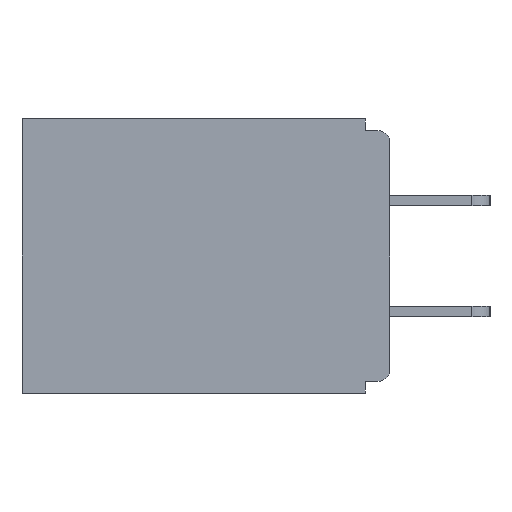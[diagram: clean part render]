
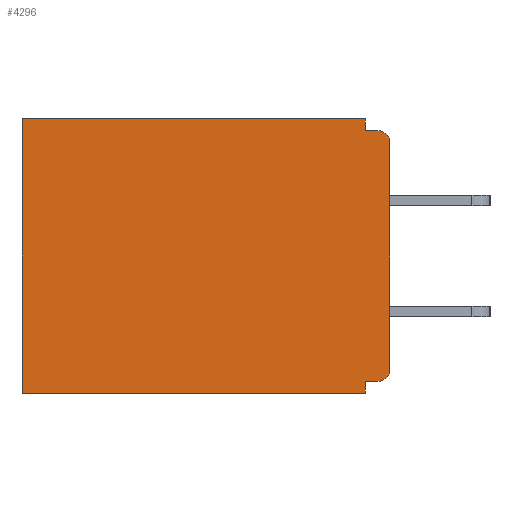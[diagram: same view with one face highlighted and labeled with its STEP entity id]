
A CAD part, left-side view. The second image highlights one B-rep face of the part: STEP entity #4296.
In plain terms, the highlighted planar face has unit normal (-1, 0, 0).
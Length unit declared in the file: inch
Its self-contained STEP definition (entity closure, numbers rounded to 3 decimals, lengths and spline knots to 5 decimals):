
#101 = CARTESIAN_POINT ( 'NONE',  ( 0.298, 0., -0.015 ) ) ;
#602 = LINE ( 'NONE', #17023, #18324 ) ;
#686 = DIRECTION ( 'NONE',  ( -1., 0., 0. ) ) ;
#735 = LINE ( 'NONE', #7220, #3177 ) ;
#1212 = EDGE_CURVE ( 'NONE', #8007, #11507, #5399, .T. ) ;
#1299 = VECTOR ( 'NONE', #16629, 39.37008 ) ;
#1311 = VERTEX_POINT ( 'NONE', #19768 ) ;
#1324 = CARTESIAN_POINT ( 'NONE',  ( 0.298, 0.031, -0.015 ) ) ;
#2215 = EDGE_CURVE ( 'NONE', #5936, #8271, #14815, .T. ) ;
#2356 = EDGE_CURVE ( 'NONE', #17014, #4807, #6064, .T. ) ;
#2443 = ORIENTED_EDGE ( 'NONE', *, *, #3839, .T. ) ;
#2468 = DIRECTION ( 'NONE',  ( 0., 1., 0. ) ) ;
#2559 = EDGE_CURVE ( 'NONE', #11507, #17014, #735, .T. ) ;
#2711 = DIRECTION ( 'NONE',  ( 1., 0., 0. ) ) ;
#2727 = CARTESIAN_POINT ( 'NONE',  ( 0.298, 0., -0.03 ) ) ;
#2842 = PLANE ( 'NONE',  #6006 ) ;
#3082 = VECTOR ( 'NONE', #13981, 39.37008 ) ;
#3177 = VECTOR ( 'NONE', #8923, 39.37008 ) ;
#3238 = ORIENTED_EDGE ( 'NONE', *, *, #1212, .F. ) ;
#3655 = ORIENTED_EDGE ( 'NONE', *, *, #2356, .F. ) ;
#3824 = AXIS2_PLACEMENT_3D ( 'NONE', #13324, #4058, #14874 ) ;
#3839 = EDGE_CURVE ( 'NONE', #8007, #1311, #12075, .T. ) ;
#4031 = CARTESIAN_POINT ( 'NONE',  ( 0.298, 0.015, -0.313 ) ) ;
#4058 = DIRECTION ( 'NONE',  ( -1., 0., 0. ) ) ;
#4099 = DIRECTION ( 'NONE',  ( 0., 1., 0. ) ) ;
#4296 = ADVANCED_FACE ( 'NONE', ( #12532 ), #2842, .F. ) ;
#4681 = EDGE_CURVE ( 'NONE', #12297, #8271, #8161, .T. ) ;
#4706 = ORIENTED_EDGE ( 'NONE', *, *, #9375, .T. ) ;
#4807 = VERTEX_POINT ( 'NONE', #15952 ) ;
#4918 = VECTOR ( 'NONE', #9161, 39.37008 ) ;
#5399 = LINE ( 'NONE', #17939, #9058 ) ;
#5936 = VERTEX_POINT ( 'NONE', #2727 ) ;
#6006 = AXIS2_PLACEMENT_3D ( 'NONE', #13664, #2711, #18236 ) ;
#6064 = LINE ( 'NONE', #10369, #15776 ) ;
#6082 = CARTESIAN_POINT ( 'NONE',  ( 0.298, 0., 0. ) ) ;
#6177 = ORIENTED_EDGE ( 'NONE', *, *, #13001, .T. ) ;
#6710 = VERTEX_POINT ( 'NONE', #19184 ) ;
#6929 = DIRECTION ( 'NONE',  ( 0., 0., -1. ) ) ;
#7220 = CARTESIAN_POINT ( 'NONE',  ( 0.298, 0.031, -0.343 ) ) ;
#7512 = CARTESIAN_POINT ( 'NONE',  ( 0.298, 0.031, -0.328 ) ) ;
#7728 = EDGE_CURVE ( 'NONE', #6710, #12297, #8160, .T. ) ;
#7798 = DIRECTION ( 'NONE',  ( 0., 1., 0. ) ) ;
#8007 = VERTEX_POINT ( 'NONE', #12739 ) ;
#8160 = LINE ( 'NONE', #18743, #3082 ) ;
#8161 = LINE ( 'NONE', #101, #15424 ) ;
#8271 = VERTEX_POINT ( 'NONE', #15710 ) ;
#8891 = AXIS2_PLACEMENT_3D ( 'NONE', #4031, #686, #6929 ) ;
#8923 = DIRECTION ( 'NONE',  ( 0., 0., -1. ) ) ;
#9058 = VECTOR ( 'NONE', #2468, 39.37008 ) ;
#9060 = LINE ( 'NONE', #6082, #4918 ) ;
#9161 = DIRECTION ( 'NONE',  ( 0., 0., -1. ) ) ;
#9237 = ORIENTED_EDGE ( 'NONE', *, *, #2559, .F. ) ;
#9301 = ORIENTED_EDGE ( 'NONE', *, *, #2215, .T. ) ;
#9375 = EDGE_CURVE ( 'NONE', #12066, #4807, #11220, .T. ) ;
#10369 = CARTESIAN_POINT ( 'NONE',  ( 0.298, 0., -0.343 ) ) ;
#11220 = LINE ( 'NONE', #18274, #1299 ) ;
#11507 = VERTEX_POINT ( 'NONE', #7512 ) ;
#12066 = VERTEX_POINT ( 'NONE', #16343 ) ;
#12075 = CIRCLE ( 'NONE', #8891, 0.015 ) ;
#12297 = VERTEX_POINT ( 'NONE', #1324 ) ;
#12532 = FACE_OUTER_BOUND ( 'NONE', #18982, .T. ) ;
#12698 = ORIENTED_EDGE ( 'NONE', *, *, #7728, .F. ) ;
#12739 = CARTESIAN_POINT ( 'NONE',  ( 0.298, 0.015, -0.328 ) ) ;
#13001 = EDGE_CURVE ( 'NONE', #6710, #12066, #602, .T. ) ;
#13324 = CARTESIAN_POINT ( 'NONE',  ( 0.298, 0.015, -0.03 ) ) ;
#13664 = CARTESIAN_POINT ( 'NONE',  ( 0.298, 0., 0. ) ) ;
#13981 = DIRECTION ( 'NONE',  ( 0., 0., -1. ) ) ;
#14020 = CARTESIAN_POINT ( 'NONE',  ( 0.298, 0.031, -0.343 ) ) ;
#14252 = EDGE_CURVE ( 'NONE', #5936, #1311, #9060, .T. ) ;
#14815 = CIRCLE ( 'NONE', #3824, 0.015 ) ;
#14874 = DIRECTION ( 'NONE',  ( 0., 0., -1. ) ) ;
#15424 = VECTOR ( 'NONE', #17191, 39.37008 ) ;
#15710 = CARTESIAN_POINT ( 'NONE',  ( 0.298, 0.015, -0.015 ) ) ;
#15776 = VECTOR ( 'NONE', #4099, 39.37008 ) ;
#15952 = CARTESIAN_POINT ( 'NONE',  ( 0.298, 0.46, -0.343 ) ) ;
#16343 = CARTESIAN_POINT ( 'NONE',  ( 0.298, 0.46, 0. ) ) ;
#16629 = DIRECTION ( 'NONE',  ( 0., 0., -1. ) ) ;
#17014 = VERTEX_POINT ( 'NONE', #14020 ) ;
#17023 = CARTESIAN_POINT ( 'NONE',  ( 0.298, 0., 0. ) ) ;
#17191 = DIRECTION ( 'NONE',  ( 0., -1., 0. ) ) ;
#17417 = ORIENTED_EDGE ( 'NONE', *, *, #14252, .F. ) ;
#17939 = CARTESIAN_POINT ( 'NONE',  ( 0.298, 0., -0.328 ) ) ;
#17964 = ORIENTED_EDGE ( 'NONE', *, *, #4681, .F. ) ;
#18236 = DIRECTION ( 'NONE',  ( 0., 0., -1. ) ) ;
#18274 = CARTESIAN_POINT ( 'NONE',  ( 0.298, 0.46, 0. ) ) ;
#18324 = VECTOR ( 'NONE', #7798, 39.37008 ) ;
#18743 = CARTESIAN_POINT ( 'NONE',  ( 0.298, 0.031, -0.343 ) ) ;
#18982 = EDGE_LOOP ( 'NONE', ( #9301, #17964, #12698, #6177, #4706, #3655, #9237, #3238, #2443, #17417 ) ) ;
#19184 = CARTESIAN_POINT ( 'NONE',  ( 0.298, 0.031, 0. ) ) ;
#19768 = CARTESIAN_POINT ( 'NONE',  ( 0.298, 0., -0.313 ) ) ;
